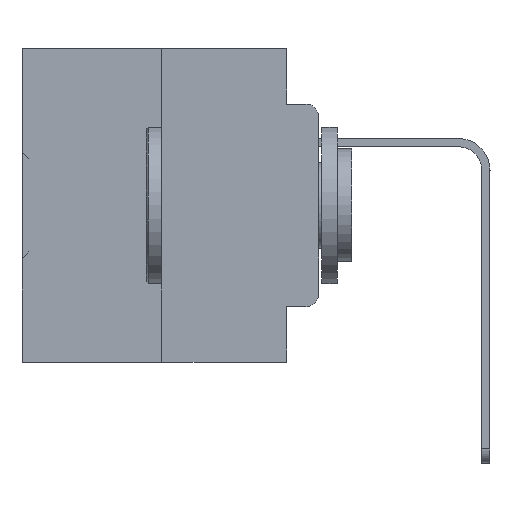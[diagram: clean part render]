
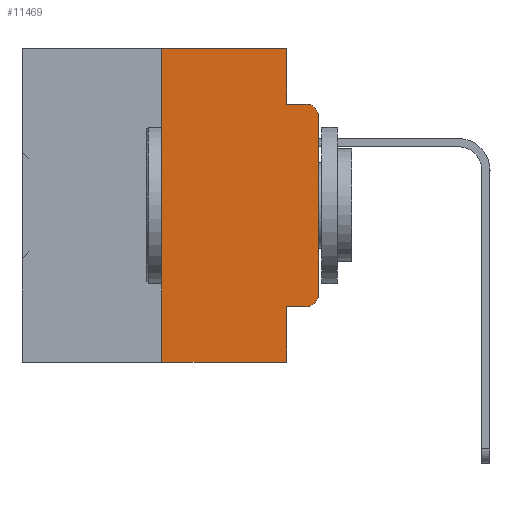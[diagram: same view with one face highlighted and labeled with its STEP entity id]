
A CAD part, left-side view. The second image highlights one B-rep face of the part: STEP entity #11469.
In plain terms, the highlighted planar face has unit normal (-1, 0, 0).
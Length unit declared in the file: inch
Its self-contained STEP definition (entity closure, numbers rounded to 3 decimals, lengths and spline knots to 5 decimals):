
#716 = DIRECTION ( 'NONE',  ( 0., -1., 0. ) ) ;
#1565 = CARTESIAN_POINT ( 'NONE',  ( 0., 0.051, 0. ) ) ;
#1646 = VECTOR ( 'NONE', #34354, 39.37008 ) ;
#2280 = CARTESIAN_POINT ( 'NONE',  ( 0., 0.02, -0.4115 ) ) ;
#2525 = CARTESIAN_POINT ( 'NONE',  ( 0., 0., 0. ) ) ;
#2568 = CARTESIAN_POINT ( 'NONE',  ( 0., 0.25, 0. ) ) ;
#2720 = CARTESIAN_POINT ( 'NONE',  ( 0., 0., -0.1085 ) ) ;
#2746 = CARTESIAN_POINT ( 'NONE',  ( 0., 0.051, -0.0885 ) ) ;
#2807 = DIRECTION ( 'NONE',  ( 0., 0., 1. ) ) ;
#3740 = VERTEX_POINT ( 'NONE', #19280 ) ;
#3877 = ORIENTED_EDGE ( 'NONE', *, *, #6616, .F. ) ;
#4120 = VECTOR ( 'NONE', #34202, 39.37008 ) ;
#4716 = CARTESIAN_POINT ( 'NONE',  ( 0., 0.473, -0.5 ) ) ;
#5547 = EDGE_CURVE ( 'NONE', #29359, #29086, #32503, .T. ) ;
#6047 = AXIS2_PLACEMENT_3D ( 'NONE', #11640, #31638, #14019 ) ;
#6101 = VERTEX_POINT ( 'NONE', #14802 ) ;
#6290 = FACE_OUTER_BOUND ( 'NONE', #13484, .T. ) ;
#6616 = EDGE_CURVE ( 'NONE', #15409, #29086, #27088, .T. ) ;
#6854 = ORIENTED_EDGE ( 'NONE', *, *, #26590, .F. ) ;
#7122 = EDGE_CURVE ( 'NONE', #23208, #29359, #25178, .T. ) ;
#8784 = CARTESIAN_POINT ( 'NONE',  ( 0., 0.051, -0.4115 ) ) ;
#9340 = AXIS2_PLACEMENT_3D ( 'NONE', #34360, #18238, #11494 ) ;
#9660 = VECTOR ( 'NONE', #716, 39.37008 ) ;
#10612 = DIRECTION ( 'NONE',  ( 0., -1., 0. ) ) ;
#11355 = CARTESIAN_POINT ( 'NONE',  ( 0., 0.051, 0. ) ) ;
#11469 = ADVANCED_FACE ( 'NONE', ( #6290 ), #28786, .F. ) ;
#11494 = DIRECTION ( 'NONE',  ( 0., 0., -1. ) ) ;
#11640 = CARTESIAN_POINT ( 'NONE',  ( 0., 0.473, 0. ) ) ;
#12305 = ORIENTED_EDGE ( 'NONE', *, *, #24117, .T. ) ;
#12327 = CARTESIAN_POINT ( 'NONE',  ( 0., 0.051, -0.4115 ) ) ;
#12896 = VECTOR ( 'NONE', #10612, 39.37008 ) ;
#12908 = VECTOR ( 'NONE', #2807, 39.37008 ) ;
#12948 = CARTESIAN_POINT ( 'NONE',  ( 0., 0.051, 0. ) ) ;
#13484 = EDGE_LOOP ( 'NONE', ( #35202, #36717, #3877, #6854, #17763, #19253, #12305, #16893, #36554, #18466 ) ) ;
#14019 = DIRECTION ( 'NONE',  ( 0., 0., -1. ) ) ;
#14802 = CARTESIAN_POINT ( 'NONE',  ( 0., 0.051, -0.5 ) ) ;
#15230 = VECTOR ( 'NONE', #18515, 39.37008 ) ;
#15409 = VERTEX_POINT ( 'NONE', #2746 ) ;
#15506 = EDGE_CURVE ( 'NONE', #17822, #34309, #25804, .T. ) ;
#16356 = DIRECTION ( 'NONE',  ( 0., -1., 0. ) ) ;
#16893 = ORIENTED_EDGE ( 'NONE', *, *, #28394, .F. ) ;
#16902 = LINE ( 'NONE', #11355, #1646 ) ;
#17031 = DIRECTION ( 'NONE',  ( 0., -1., 0. ) ) ;
#17467 = EDGE_CURVE ( 'NONE', #3740, #21648, #35017, .T. ) ;
#17668 = CARTESIAN_POINT ( 'NONE',  ( 0., 0.02, -0.0885 ) ) ;
#17763 = ORIENTED_EDGE ( 'NONE', *, *, #17467, .F. ) ;
#17822 = VERTEX_POINT ( 'NONE', #12327 ) ;
#18238 = DIRECTION ( 'NONE',  ( -1., 0., 0. ) ) ;
#18466 = ORIENTED_EDGE ( 'NONE', *, *, #29224, .T. ) ;
#18515 = DIRECTION ( 'NONE',  ( 0., 0., -1. ) ) ;
#19253 = ORIENTED_EDGE ( 'NONE', *, *, #35631, .F. ) ;
#19280 = CARTESIAN_POINT ( 'NONE',  ( 0., 0.25, 0. ) ) ;
#20506 = CARTESIAN_POINT ( 'NONE',  ( 0., 0.25, -0.5 ) ) ;
#21380 = CIRCLE ( 'NONE', #24832, 0.02 ) ;
#21648 = VERTEX_POINT ( 'NONE', #12948 ) ;
#22192 = CARTESIAN_POINT ( 'NONE',  ( 0., 0.02, -0.3915 ) ) ;
#23208 = VERTEX_POINT ( 'NONE', #33934 ) ;
#23765 = LINE ( 'NONE', #1565, #15230 ) ;
#24117 = EDGE_CURVE ( 'NONE', #33929, #6101, #33927, .T. ) ;
#24832 = AXIS2_PLACEMENT_3D ( 'NONE', #22192, #35695, #35432 ) ;
#24980 = CARTESIAN_POINT ( 'NONE',  ( 0., 0.473, 0. ) ) ;
#25178 = LINE ( 'NONE', #2525, #4120 ) ;
#25804 = LINE ( 'NONE', #8784, #9660 ) ;
#26590 = EDGE_CURVE ( 'NONE', #21648, #15409, #23765, .T. ) ;
#26997 = VECTOR ( 'NONE', #16356, 39.37008 ) ;
#27088 = LINE ( 'NONE', #28802, #32862 ) ;
#28394 = EDGE_CURVE ( 'NONE', #17822, #6101, #16902, .T. ) ;
#28786 = PLANE ( 'NONE',  #6047 ) ;
#28802 = CARTESIAN_POINT ( 'NONE',  ( 0., 0.051, -0.0885 ) ) ;
#29086 = VERTEX_POINT ( 'NONE', #17668 ) ;
#29224 = EDGE_CURVE ( 'NONE', #34309, #23208, #21380, .T. ) ;
#29359 = VERTEX_POINT ( 'NONE', #2720 ) ;
#31638 = DIRECTION ( 'NONE',  ( 1., 0., 0. ) ) ;
#32503 = CIRCLE ( 'NONE', #9340, 0.02 ) ;
#32862 = VECTOR ( 'NONE', #17031, 39.37008 ) ;
#33927 = LINE ( 'NONE', #4716, #12896 ) ;
#33929 = VERTEX_POINT ( 'NONE', #20506 ) ;
#33934 = CARTESIAN_POINT ( 'NONE',  ( 0., 0., -0.3915 ) ) ;
#34202 = DIRECTION ( 'NONE',  ( 0., 0., 1. ) ) ;
#34309 = VERTEX_POINT ( 'NONE', #2280 ) ;
#34354 = DIRECTION ( 'NONE',  ( 0., 0., -1. ) ) ;
#34360 = CARTESIAN_POINT ( 'NONE',  ( 0., 0.02, -0.1085 ) ) ;
#34400 = LINE ( 'NONE', #2568, #12908 ) ;
#35017 = LINE ( 'NONE', #24980, #26997 ) ;
#35202 = ORIENTED_EDGE ( 'NONE', *, *, #7122, .T. ) ;
#35432 = DIRECTION ( 'NONE',  ( 0., 0., -1. ) ) ;
#35631 = EDGE_CURVE ( 'NONE', #33929, #3740, #34400, .T. ) ;
#35695 = DIRECTION ( 'NONE',  ( -1., 0., 0. ) ) ;
#36554 = ORIENTED_EDGE ( 'NONE', *, *, #15506, .T. ) ;
#36717 = ORIENTED_EDGE ( 'NONE', *, *, #5547, .T. ) ;
